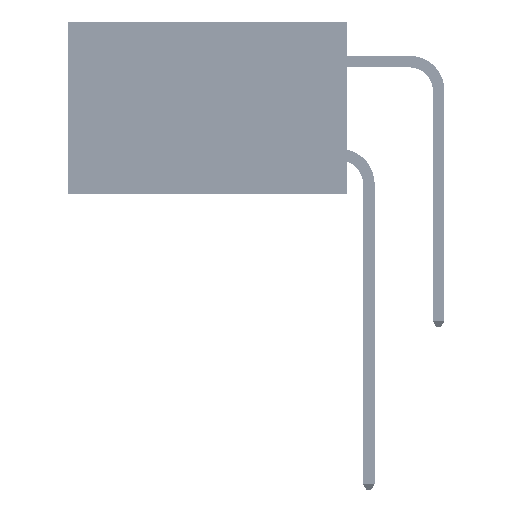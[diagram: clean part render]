
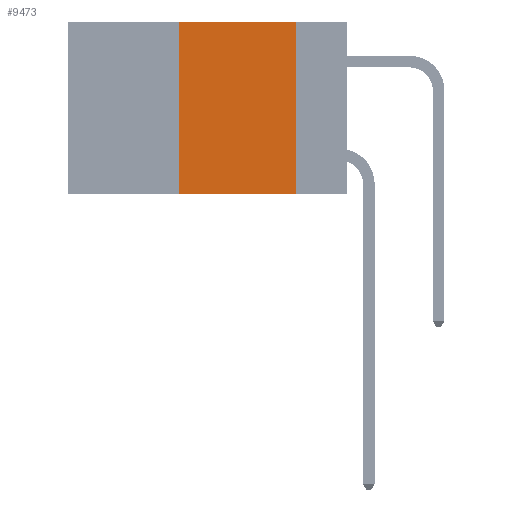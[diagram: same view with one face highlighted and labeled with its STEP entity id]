
A CAD part, left-side view. The second image highlights one B-rep face of the part: STEP entity #9473.
In plain terms, the highlighted planar face has unit normal (-1, 0, 0).
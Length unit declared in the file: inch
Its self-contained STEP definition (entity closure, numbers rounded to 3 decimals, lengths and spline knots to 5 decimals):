
#225 = DIRECTION ( 'NONE',  ( 0., -1., 0. ) ) ;
#2170 = CARTESIAN_POINT ( 'NONE',  ( 0., 0.6, 0. ) ) ;
#5401 = LINE ( 'NONE', #20647, #33538 ) ;
#5432 = EDGE_CURVE ( 'NONE', #28253, #33055, #10677, .T. ) ;
#6577 = CARTESIAN_POINT ( 'NONE',  ( 0., 0.36, -0.37 ) ) ;
#7824 = FACE_OUTER_BOUND ( 'NONE', #9094, .T. ) ;
#9091 = LINE ( 'NONE', #25247, #44872 ) ;
#9094 = EDGE_LOOP ( 'NONE', ( #18390, #14348, #34785, #33173 ) ) ;
#9473 = ADVANCED_FACE ( 'NONE', ( #7824 ), #9556, .F. ) ;
#9556 = PLANE ( 'NONE',  #27632 ) ;
#10677 = LINE ( 'NONE', #30986, #47813 ) ;
#13289 = VECTOR ( 'NONE', #22152, 39.37008 ) ;
#14348 = ORIENTED_EDGE ( 'NONE', *, *, #20011, .F. ) ;
#17230 = EDGE_CURVE ( 'NONE', #28253, #18274, #38250, .T. ) ;
#17943 = DIRECTION ( 'NONE',  ( 0., 0., -1. ) ) ;
#18274 = VERTEX_POINT ( 'NONE', #38218 ) ;
#18390 = ORIENTED_EDGE ( 'NONE', *, *, #29206, .F. ) ;
#20011 = EDGE_CURVE ( 'NONE', #33055, #34835, #5401, .T. ) ;
#20647 = CARTESIAN_POINT ( 'NONE',  ( 0., 0.6, 0. ) ) ;
#21198 = CARTESIAN_POINT ( 'NONE',  ( 0., 0.36, 0. ) ) ;
#21889 = DIRECTION ( 'NONE',  ( 1., 0., 0. ) ) ;
#22152 = DIRECTION ( 'NONE',  ( 0., -1., 0. ) ) ;
#25247 = CARTESIAN_POINT ( 'NONE',  ( 0., 0.11, 0. ) ) ;
#26891 = DIRECTION ( 'NONE',  ( 0., 0., 1. ) ) ;
#27632 = AXIS2_PLACEMENT_3D ( 'NONE', #2170, #21889, #17943 ) ;
#28253 = VERTEX_POINT ( 'NONE', #6577 ) ;
#29206 = EDGE_CURVE ( 'NONE', #34835, #18274, #9091, .T. ) ;
#30986 = CARTESIAN_POINT ( 'NONE',  ( 0., 0.36, 0. ) ) ;
#33055 = VERTEX_POINT ( 'NONE', #21198 ) ;
#33173 = ORIENTED_EDGE ( 'NONE', *, *, #17230, .T. ) ;
#33538 = VECTOR ( 'NONE', #225, 39.37008 ) ;
#34785 = ORIENTED_EDGE ( 'NONE', *, *, #5432, .F. ) ;
#34835 = VERTEX_POINT ( 'NONE', #52784 ) ;
#38218 = CARTESIAN_POINT ( 'NONE',  ( 0., 0.11, -0.37 ) ) ;
#38250 = LINE ( 'NONE', #51120, #13289 ) ;
#44872 = VECTOR ( 'NONE', #50084, 39.37008 ) ;
#47813 = VECTOR ( 'NONE', #26891, 39.37008 ) ;
#50084 = DIRECTION ( 'NONE',  ( 0., 0., -1. ) ) ;
#51120 = CARTESIAN_POINT ( 'NONE',  ( 0., 0.6, -0.37 ) ) ;
#52784 = CARTESIAN_POINT ( 'NONE',  ( 0., 0.11, 0. ) ) ;
